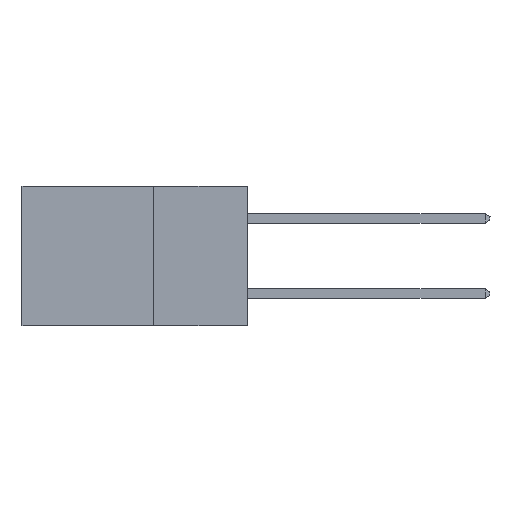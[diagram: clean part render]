
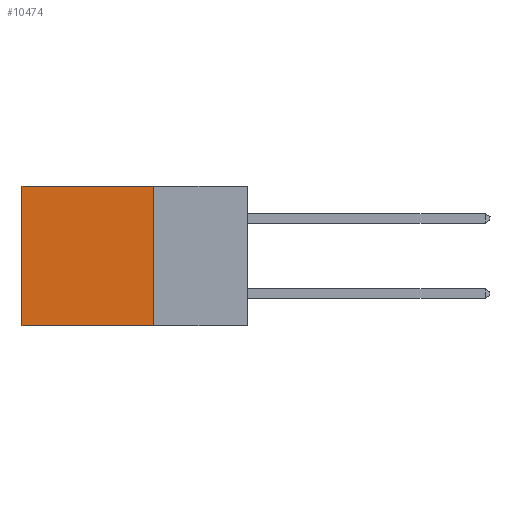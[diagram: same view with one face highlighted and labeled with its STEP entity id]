
A CAD part, left-side view. The second image highlights one B-rep face of the part: STEP entity #10474.
In plain terms, the highlighted planar face has unit normal (-1, 0, 0).
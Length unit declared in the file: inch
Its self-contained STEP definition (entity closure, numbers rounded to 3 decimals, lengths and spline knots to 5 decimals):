
#1074 = DIRECTION ( 'NONE',  ( 0., 1., 0. ) ) ;
#1268 = VERTEX_POINT ( 'NONE', #18710 ) ;
#1679 = ORIENTED_EDGE ( 'NONE', *, *, #8288, .F. ) ;
#1998 = VERTEX_POINT ( 'NONE', #10242 ) ;
#6188 = VECTOR ( 'NONE', #1074, 39.37008 ) ;
#7752 = CARTESIAN_POINT ( 'NONE',  ( 0.298, 0.25, -0.37 ) ) ;
#8288 = EDGE_CURVE ( 'NONE', #1998, #1268, #26539, .T. ) ;
#8460 = EDGE_CURVE ( 'NONE', #15094, #1268, #18600, .T. ) ;
#8914 = CARTESIAN_POINT ( 'NONE',  ( 0.298, 0.6, 0. ) ) ;
#8946 = VECTOR ( 'NONE', #23657, 39.37008 ) ;
#9034 = PLANE ( 'NONE',  #27427 ) ;
#9673 = DIRECTION ( 'NONE',  ( 1., 0., 0. ) ) ;
#10242 = CARTESIAN_POINT ( 'NONE',  ( 0.298, 0.25, -0.37 ) ) ;
#10474 = ADVANCED_FACE ( 'NONE', ( #17491 ), #9034, .F. ) ;
#10548 = CARTESIAN_POINT ( 'NONE',  ( 0.298, 0.25, 0. ) ) ;
#14096 = ORIENTED_EDGE ( 'NONE', *, *, #21535, .T. ) ;
#14549 = DIRECTION ( 'NONE',  ( 0., 0., -1. ) ) ;
#15094 = VERTEX_POINT ( 'NONE', #15337 ) ;
#15142 = LINE ( 'NONE', #27364, #19617 ) ;
#15337 = CARTESIAN_POINT ( 'NONE',  ( 0.298, 0.6, 0. ) ) ;
#15367 = EDGE_LOOP ( 'NONE', ( #18449, #1679, #23689, #14096 ) ) ;
#15387 = DIRECTION ( 'NONE',  ( 0., 1., 0. ) ) ;
#15433 = DIRECTION ( 'NONE',  ( 0., 0., -1. ) ) ;
#17491 = FACE_OUTER_BOUND ( 'NONE', #15367, .T. ) ;
#18012 = CARTESIAN_POINT ( 'NONE',  ( 0.298, 0.25, 0. ) ) ;
#18449 = ORIENTED_EDGE ( 'NONE', *, *, #8460, .T. ) ;
#18600 = LINE ( 'NONE', #8914, #8946 ) ;
#18710 = CARTESIAN_POINT ( 'NONE',  ( 0.298, 0.6, -0.37 ) ) ;
#19617 = VECTOR ( 'NONE', #14549, 39.37008 ) ;
#20219 = CARTESIAN_POINT ( 'NONE',  ( 0.298, 0.25, 0. ) ) ;
#20574 = VECTOR ( 'NONE', #15387, 39.37008 ) ;
#21535 = EDGE_CURVE ( 'NONE', #25946, #15094, #26744, .T. ) ;
#23657 = DIRECTION ( 'NONE',  ( 0., 0., -1. ) ) ;
#23689 = ORIENTED_EDGE ( 'NONE', *, *, #26323, .F. ) ;
#25946 = VERTEX_POINT ( 'NONE', #20219 ) ;
#26323 = EDGE_CURVE ( 'NONE', #25946, #1998, #15142, .T. ) ;
#26539 = LINE ( 'NONE', #7752, #6188 ) ;
#26744 = LINE ( 'NONE', #10548, #20574 ) ;
#27364 = CARTESIAN_POINT ( 'NONE',  ( 0.298, 0.25, 0. ) ) ;
#27427 = AXIS2_PLACEMENT_3D ( 'NONE', #18012, #9673, #15433 ) ;
